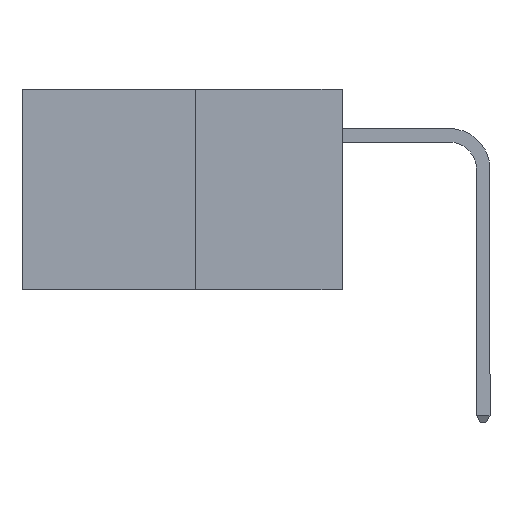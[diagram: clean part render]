
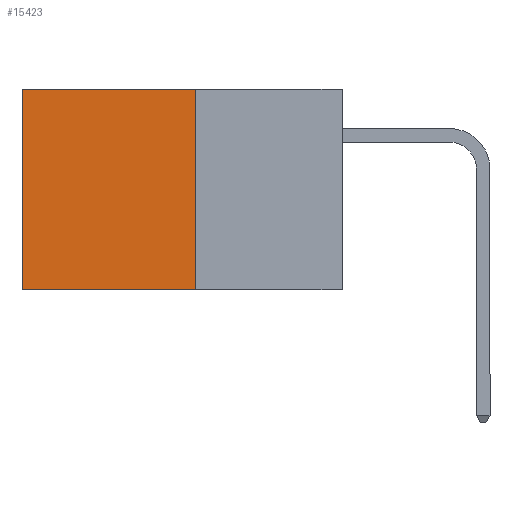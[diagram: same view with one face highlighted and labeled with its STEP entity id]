
A CAD part, left-side view. The second image highlights one B-rep face of the part: STEP entity #15423.
In plain terms, the highlighted planar face has unit normal (-1, 0, 0).
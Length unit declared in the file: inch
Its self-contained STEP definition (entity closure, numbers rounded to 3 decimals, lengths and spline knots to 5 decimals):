
#891 = CARTESIAN_POINT ( 'NONE',  ( 0.277, 0.59, -0.37 ) ) ;
#1109 = EDGE_LOOP ( 'NONE', ( #20660, #4605, #12560, #23362 ) ) ;
#1831 = LINE ( 'NONE', #891, #12578 ) ;
#2394 = AXIS2_PLACEMENT_3D ( 'NONE', #17823, #11598, #26128 ) ;
#3098 = CARTESIAN_POINT ( 'NONE',  ( 0.277, 0.27, -0.37 ) ) ;
#3675 = DIRECTION ( 'NONE',  ( 0., 0., -1. ) ) ;
#3939 = EDGE_CURVE ( 'NONE', #9836, #9583, #1831, .T. ) ;
#4243 = CARTESIAN_POINT ( 'NONE',  ( 0.277, 0.27, -0.37 ) ) ;
#4605 = ORIENTED_EDGE ( 'NONE', *, *, #21169, .F. ) ;
#5090 = CARTESIAN_POINT ( 'NONE',  ( 0.277, 0.27, 0. ) ) ;
#7460 = VERTEX_POINT ( 'NONE', #15894 ) ;
#7977 = CARTESIAN_POINT ( 'NONE',  ( 0.277, 0.59, -0.37 ) ) ;
#8642 = DIRECTION ( 'NONE',  ( 0., 1., 0. ) ) ;
#9500 = PLANE ( 'NONE',  #2394 ) ;
#9583 = VERTEX_POINT ( 'NONE', #7977 ) ;
#9638 = DIRECTION ( 'NONE',  ( 0., 0., -1. ) ) ;
#9836 = VERTEX_POINT ( 'NONE', #25511 ) ;
#10838 = VECTOR ( 'NONE', #8642, 39.37008 ) ;
#11587 = DIRECTION ( 'NONE',  ( 0., 1., 0. ) ) ;
#11598 = DIRECTION ( 'NONE',  ( 1., 0., 0. ) ) ;
#12560 = ORIENTED_EDGE ( 'NONE', *, *, #13884, .F. ) ;
#12578 = VECTOR ( 'NONE', #9638, 39.37008 ) ;
#12758 = VERTEX_POINT ( 'NONE', #3098 ) ;
#13884 = EDGE_CURVE ( 'NONE', #7460, #12758, #24519, .T. ) ;
#14382 = CARTESIAN_POINT ( 'NONE',  ( 0.277, 0.27, -0.37 ) ) ;
#14715 = VECTOR ( 'NONE', #11587, 39.37008 ) ;
#15423 = ADVANCED_FACE ( 'NONE', ( #22807 ), #9500, .F. ) ;
#15894 = CARTESIAN_POINT ( 'NONE',  ( 0.277, 0.27, 0. ) ) ;
#16374 = LINE ( 'NONE', #4243, #10838 ) ;
#17823 = CARTESIAN_POINT ( 'NONE',  ( 0.277, 0.27, -0.37 ) ) ;
#20660 = ORIENTED_EDGE ( 'NONE', *, *, #3939, .T. ) ;
#21169 = EDGE_CURVE ( 'NONE', #12758, #9583, #16374, .T. ) ;
#21415 = EDGE_CURVE ( 'NONE', #7460, #9836, #25770, .T. ) ;
#22807 = FACE_OUTER_BOUND ( 'NONE', #1109, .T. ) ;
#23362 = ORIENTED_EDGE ( 'NONE', *, *, #21415, .T. ) ;
#23873 = VECTOR ( 'NONE', #3675, 39.37008 ) ;
#24519 = LINE ( 'NONE', #14382, #23873 ) ;
#25511 = CARTESIAN_POINT ( 'NONE',  ( 0.277, 0.59, 0. ) ) ;
#25770 = LINE ( 'NONE', #5090, #14715 ) ;
#26128 = DIRECTION ( 'NONE',  ( 0., 0., -1. ) ) ;
